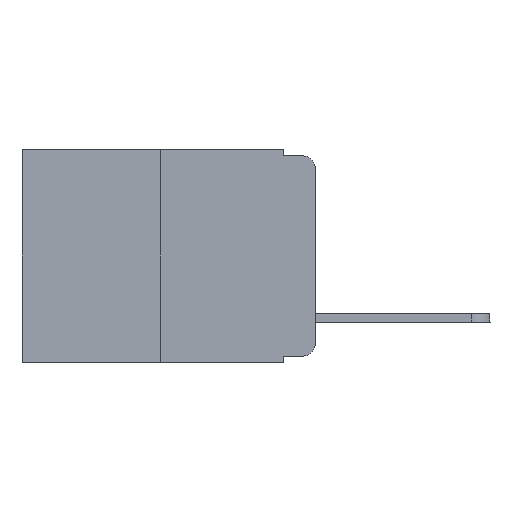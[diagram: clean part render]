
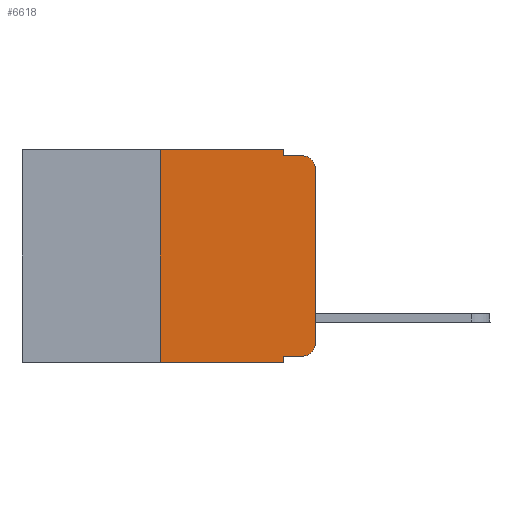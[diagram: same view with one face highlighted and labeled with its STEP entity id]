
A CAD part, left-side view. The second image highlights one B-rep face of the part: STEP entity #6618.
In plain terms, the highlighted planar face has unit normal (-1, 0, 0).
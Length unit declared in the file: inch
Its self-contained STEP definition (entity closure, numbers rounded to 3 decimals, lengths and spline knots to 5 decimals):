
#359 = ORIENTED_EDGE ( 'NONE', *, *, #12040, .T. ) ;
#678 = DIRECTION ( 'NONE',  ( 0., 0., -1. ) ) ;
#731 = VECTOR ( 'NONE', #13051, 39.37008 ) ;
#746 = LINE ( 'NONE', #1645, #13030 ) ;
#794 = AXIS2_PLACEMENT_3D ( 'NONE', #1750, #10022, #6497 ) ;
#870 = CARTESIAN_POINT ( 'NONE',  ( 0., 0.25, -0.343 ) ) ;
#1619 = VECTOR ( 'NONE', #9863, 39.37008 ) ;
#1641 = VERTEX_POINT ( 'NONE', #8889 ) ;
#1645 = CARTESIAN_POINT ( 'NONE',  ( 0., 0., 0. ) ) ;
#1650 = VERTEX_POINT ( 'NONE', #4098 ) ;
#1669 = VECTOR ( 'NONE', #12824, 39.37008 ) ;
#1750 = CARTESIAN_POINT ( 'NONE',  ( 0., 0.02, -0.313 ) ) ;
#2023 = LINE ( 'NONE', #6683, #3695 ) ;
#2137 = ORIENTED_EDGE ( 'NONE', *, *, #12494, .F. ) ;
#2464 = CARTESIAN_POINT ( 'NONE',  ( 0., 0.051, 0. ) ) ;
#2776 = ORIENTED_EDGE ( 'NONE', *, *, #10035, .T. ) ;
#2834 = PLANE ( 'NONE',  #10950 ) ;
#3099 = CARTESIAN_POINT ( 'NONE',  ( 0., 0., -0.03 ) ) ;
#3173 = VERTEX_POINT ( 'NONE', #8727 ) ;
#3639 = ORIENTED_EDGE ( 'NONE', *, *, #7966, .T. ) ;
#3695 = VECTOR ( 'NONE', #5527, 39.37008 ) ;
#3713 = VERTEX_POINT ( 'NONE', #14700 ) ;
#4098 = CARTESIAN_POINT ( 'NONE',  ( 0., 0.02, -0.01 ) ) ;
#4519 = CARTESIAN_POINT ( 'NONE',  ( 0., 0.051, 0. ) ) ;
#4713 = ORIENTED_EDGE ( 'NONE', *, *, #14604, .F. ) ;
#4941 = VECTOR ( 'NONE', #8565, 39.37008 ) ;
#5068 = CIRCLE ( 'NONE', #794, 0.02 ) ;
#5272 = EDGE_LOOP ( 'NONE', ( #359, #13761, #4713, #11400, #2137, #7734, #2776, #9186, #3639, #9814 ) ) ;
#5340 = VERTEX_POINT ( 'NONE', #3099 ) ;
#5385 = VERTEX_POINT ( 'NONE', #6912 ) ;
#5527 = DIRECTION ( 'NONE',  ( 0., 0., 1. ) ) ;
#5560 = LINE ( 'NONE', #12898, #731 ) ;
#5642 = VERTEX_POINT ( 'NONE', #7413 ) ;
#6159 = VERTEX_POINT ( 'NONE', #2464 ) ;
#6497 = DIRECTION ( 'NONE',  ( 0., 0., -1. ) ) ;
#6618 = ADVANCED_FACE ( 'NONE', ( #9263 ), #2834, .F. ) ;
#6683 = CARTESIAN_POINT ( 'NONE',  ( 0., 0.25, 0. ) ) ;
#6888 = DIRECTION ( 'NONE',  ( 0., -1., 0. ) ) ;
#6912 = CARTESIAN_POINT ( 'NONE',  ( 0., 0.051, -0.343 ) ) ;
#7260 = EDGE_CURVE ( 'NONE', #10217, #5642, #2023, .T. ) ;
#7413 = CARTESIAN_POINT ( 'NONE',  ( 0., 0.25, 0. ) ) ;
#7454 = CARTESIAN_POINT ( 'NONE',  ( 0., 0.473, -0.343 ) ) ;
#7573 = DIRECTION ( 'NONE',  ( -1., 0., 0. ) ) ;
#7689 = LINE ( 'NONE', #14716, #1619 ) ;
#7734 = ORIENTED_EDGE ( 'NONE', *, *, #7260, .F. ) ;
#7773 = CARTESIAN_POINT ( 'NONE',  ( 0., 0.051, 0. ) ) ;
#7966 = EDGE_CURVE ( 'NONE', #13312, #1641, #15394, .T. ) ;
#8247 = CARTESIAN_POINT ( 'NONE',  ( 0., 0.051, -0.333 ) ) ;
#8328 = LINE ( 'NONE', #4519, #1669 ) ;
#8486 = CIRCLE ( 'NONE', #13497, 0.02 ) ;
#8565 = DIRECTION ( 'NONE',  ( 0., -1., 0. ) ) ;
#8612 = LINE ( 'NONE', #7454, #4941 ) ;
#8651 = LINE ( 'NONE', #7773, #9772 ) ;
#8671 = DIRECTION ( 'NONE',  ( 0., 0., 1. ) ) ;
#8727 = CARTESIAN_POINT ( 'NONE',  ( 0., 0.051, -0.01 ) ) ;
#8841 = VECTOR ( 'NONE', #6888, 39.37008 ) ;
#8889 = CARTESIAN_POINT ( 'NONE',  ( 0., 0.02, -0.333 ) ) ;
#9186 = ORIENTED_EDGE ( 'NONE', *, *, #14116, .F. ) ;
#9263 = FACE_OUTER_BOUND ( 'NONE', #5272, .T. ) ;
#9772 = VECTOR ( 'NONE', #678, 39.37008 ) ;
#9814 = ORIENTED_EDGE ( 'NONE', *, *, #11282, .T. ) ;
#9833 = CARTESIAN_POINT ( 'NONE',  ( 0., 0.051, -0.333 ) ) ;
#9863 = DIRECTION ( 'NONE',  ( 0., -1., 0. ) ) ;
#10022 = DIRECTION ( 'NONE',  ( -1., 0., 0. ) ) ;
#10035 = EDGE_CURVE ( 'NONE', #10217, #5385, #8612, .T. ) ;
#10066 = DIRECTION ( 'NONE',  ( 0., 0., -1. ) ) ;
#10217 = VERTEX_POINT ( 'NONE', #870 ) ;
#10950 = AXIS2_PLACEMENT_3D ( 'NONE', #14631, #12388, #14723 ) ;
#11282 = EDGE_CURVE ( 'NONE', #1641, #3713, #5068, .T. ) ;
#11400 = ORIENTED_EDGE ( 'NONE', *, *, #13041, .F. ) ;
#12040 = EDGE_CURVE ( 'NONE', #3713, #5340, #746, .T. ) ;
#12388 = DIRECTION ( 'NONE',  ( 1., 0., 0. ) ) ;
#12494 = EDGE_CURVE ( 'NONE', #5642, #6159, #5560, .T. ) ;
#12824 = DIRECTION ( 'NONE',  ( 0., 0., -1. ) ) ;
#12898 = CARTESIAN_POINT ( 'NONE',  ( 0., 0.473, 0. ) ) ;
#13030 = VECTOR ( 'NONE', #8671, 39.37008 ) ;
#13041 = EDGE_CURVE ( 'NONE', #6159, #3173, #8328, .T. ) ;
#13051 = DIRECTION ( 'NONE',  ( 0., -1., 0. ) ) ;
#13312 = VERTEX_POINT ( 'NONE', #9833 ) ;
#13497 = AXIS2_PLACEMENT_3D ( 'NONE', #14725, #7573, #10066 ) ;
#13761 = ORIENTED_EDGE ( 'NONE', *, *, #13896, .T. ) ;
#13896 = EDGE_CURVE ( 'NONE', #5340, #1650, #8486, .T. ) ;
#14116 = EDGE_CURVE ( 'NONE', #13312, #5385, #8651, .T. ) ;
#14604 = EDGE_CURVE ( 'NONE', #3173, #1650, #7689, .T. ) ;
#14631 = CARTESIAN_POINT ( 'NONE',  ( 0., 0.473, 0. ) ) ;
#14700 = CARTESIAN_POINT ( 'NONE',  ( 0., 0., -0.313 ) ) ;
#14716 = CARTESIAN_POINT ( 'NONE',  ( 0., 0.051, -0.01 ) ) ;
#14723 = DIRECTION ( 'NONE',  ( 0., 0., -1. ) ) ;
#14725 = CARTESIAN_POINT ( 'NONE',  ( 0., 0.02, -0.03 ) ) ;
#15394 = LINE ( 'NONE', #8247, #8841 ) ;
